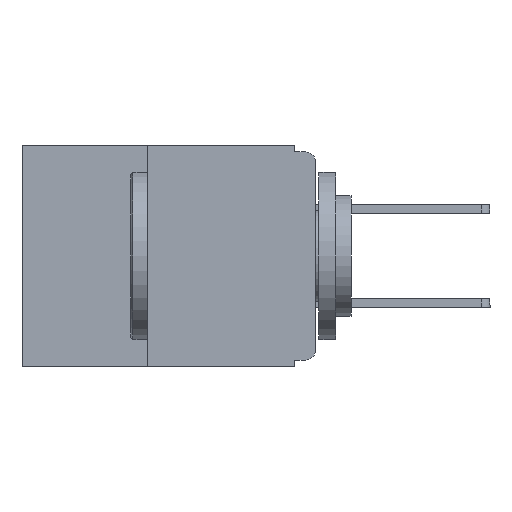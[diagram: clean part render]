
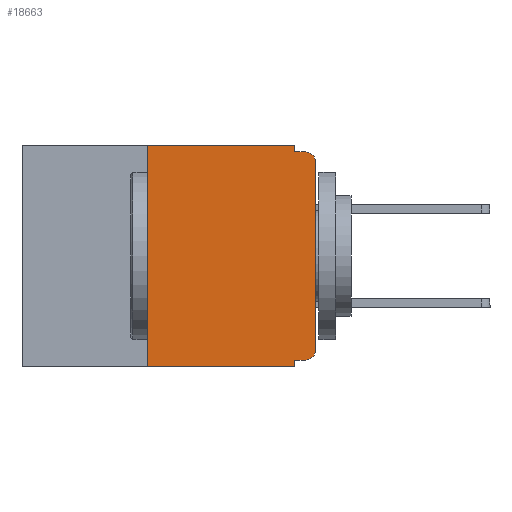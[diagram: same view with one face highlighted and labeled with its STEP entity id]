
A CAD part, left-side view. The second image highlights one B-rep face of the part: STEP entity #18663.
In plain terms, the highlighted planar face has unit normal (-1, 0, 0).
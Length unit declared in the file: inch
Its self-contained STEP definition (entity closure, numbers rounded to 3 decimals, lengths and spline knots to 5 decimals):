
#309 = EDGE_CURVE ( 'NONE', #14362, #420, #9314, .T. ) ;
#420 = VERTEX_POINT ( 'NONE', #20970 ) ;
#1340 = EDGE_CURVE ( 'NONE', #6322, #14299, #17589, .T. ) ;
#1489 = VERTEX_POINT ( 'NONE', #14184 ) ;
#2234 = ORIENTED_EDGE ( 'NONE', *, *, #12778, .T. ) ;
#2602 = ORIENTED_EDGE ( 'NONE', *, *, #5748, .F. ) ;
#2698 = ORIENTED_EDGE ( 'NONE', *, *, #8551, .T. ) ;
#2961 = CARTESIAN_POINT ( 'NONE',  ( 0., 0., -0.01 ) ) ;
#3561 = CARTESIAN_POINT ( 'NONE',  ( 0., 0.031, -0.01 ) ) ;
#3616 = VECTOR ( 'NONE', #21447, 39.37008 ) ;
#3746 = VERTEX_POINT ( 'NONE', #11124 ) ;
#4279 = ORIENTED_EDGE ( 'NONE', *, *, #15386, .T. ) ;
#4288 = ORIENTED_EDGE ( 'NONE', *, *, #10600, .F. ) ;
#4290 = LINE ( 'NONE', #2961, #12814 ) ;
#4344 = CARTESIAN_POINT ( 'NONE',  ( 0., 0., -0.32 ) ) ;
#4384 = DIRECTION ( 'NONE',  ( 0., 0., -1. ) ) ;
#4617 = VERTEX_POINT ( 'NONE', #19635 ) ;
#4708 = DIRECTION ( 'NONE',  ( 0., -1., 0. ) ) ;
#5220 = DIRECTION ( 'NONE',  ( 0., -1., 0. ) ) ;
#5565 = VECTOR ( 'NONE', #5220, 39.37008 ) ;
#5639 = DIRECTION ( 'NONE',  ( 0., 1., 0. ) ) ;
#5748 = EDGE_CURVE ( 'NONE', #3746, #12291, #14736, .T. ) ;
#6243 = DIRECTION ( 'NONE',  ( 0., 0., 1. ) ) ;
#6317 = PLANE ( 'NONE',  #16685 ) ;
#6322 = VERTEX_POINT ( 'NONE', #11611 ) ;
#6332 = CARTESIAN_POINT ( 'NONE',  ( 0., 0., 0. ) ) ;
#6452 = DIRECTION ( 'NONE',  ( 0., -1., 0. ) ) ;
#6865 = LINE ( 'NONE', #4344, #11410 ) ;
#7360 = EDGE_LOOP ( 'NONE', ( #2234, #2698, #13520, #14087, #4288, #2602, #4279, #10734, #19033, #18287 ) ) ;
#8551 = EDGE_CURVE ( 'NONE', #4617, #1489, #9394, .T. ) ;
#8654 = CARTESIAN_POINT ( 'NONE',  ( 0., 0.031, 0. ) ) ;
#9064 = LINE ( 'NONE', #8654, #17898 ) ;
#9314 = CIRCLE ( 'NONE', #10658, 0.015 ) ;
#9394 = CIRCLE ( 'NONE', #10488, 0.015 ) ;
#9751 = DIRECTION ( 'NONE',  ( 1., 0., 0. ) ) ;
#10041 = CARTESIAN_POINT ( 'NONE',  ( 0., 0.031, -0.33 ) ) ;
#10049 = VERTEX_POINT ( 'NONE', #3561 ) ;
#10380 = DIRECTION ( 'NONE',  ( 0., 0., -1. ) ) ;
#10488 = AXIS2_PLACEMENT_3D ( 'NONE', #18037, #18027, #17991 ) ;
#10600 = EDGE_CURVE ( 'NONE', #12291, #19968, #15083, .T. ) ;
#10658 = AXIS2_PLACEMENT_3D ( 'NONE', #21500, #12845, #4384 ) ;
#10734 = ORIENTED_EDGE ( 'NONE', *, *, #1340, .F. ) ;
#11124 = CARTESIAN_POINT ( 'NONE',  ( 0., 0.25, -0.33 ) ) ;
#11225 = EDGE_CURVE ( 'NONE', #14362, #6322, #6865, .T. ) ;
#11379 = VECTOR ( 'NONE', #6243, 39.37008 ) ;
#11410 = VECTOR ( 'NONE', #5639, 39.37008 ) ;
#11588 = CARTESIAN_POINT ( 'NONE',  ( 0., 0.25, 0. ) ) ;
#11611 = CARTESIAN_POINT ( 'NONE',  ( 0., 0.031, -0.32 ) ) ;
#11764 = VECTOR ( 'NONE', #6452, 39.37008 ) ;
#11915 = FACE_OUTER_BOUND ( 'NONE', #7360, .T. ) ;
#12291 = VERTEX_POINT ( 'NONE', #11588 ) ;
#12778 = EDGE_CURVE ( 'NONE', #420, #4617, #15812, .T. ) ;
#12814 = VECTOR ( 'NONE', #4708, 39.37008 ) ;
#12845 = DIRECTION ( 'NONE',  ( -1., 0., 0. ) ) ;
#13343 = CARTESIAN_POINT ( 'NONE',  ( 0., 0.437, -0.33 ) ) ;
#13520 = ORIENTED_EDGE ( 'NONE', *, *, #15347, .F. ) ;
#14087 = ORIENTED_EDGE ( 'NONE', *, *, #17657, .F. ) ;
#14184 = CARTESIAN_POINT ( 'NONE',  ( 0., 0.015, -0.01 ) ) ;
#14299 = VERTEX_POINT ( 'NONE', #20276 ) ;
#14362 = VERTEX_POINT ( 'NONE', #15627 ) ;
#14391 = CARTESIAN_POINT ( 'NONE',  ( 0., 0.031, 0. ) ) ;
#14736 = LINE ( 'NONE', #17342, #18551 ) ;
#15083 = LINE ( 'NONE', #15618, #5565 ) ;
#15347 = EDGE_CURVE ( 'NONE', #10049, #1489, #4290, .T. ) ;
#15386 = EDGE_CURVE ( 'NONE', #3746, #14299, #21446, .T. ) ;
#15618 = CARTESIAN_POINT ( 'NONE',  ( 0., 0.437, 0. ) ) ;
#15627 = CARTESIAN_POINT ( 'NONE',  ( 0., 0.015, -0.32 ) ) ;
#15812 = LINE ( 'NONE', #6332, #11379 ) ;
#16685 = AXIS2_PLACEMENT_3D ( 'NONE', #18002, #9751, #21202 ) ;
#17342 = CARTESIAN_POINT ( 'NONE',  ( 0., 0.25, -0.33 ) ) ;
#17365 = DIRECTION ( 'NONE',  ( 0., 0., 1. ) ) ;
#17589 = LINE ( 'NONE', #10041, #3616 ) ;
#17657 = EDGE_CURVE ( 'NONE', #19968, #10049, #9064, .T. ) ;
#17898 = VECTOR ( 'NONE', #10380, 39.37008 ) ;
#17991 = DIRECTION ( 'NONE',  ( 0., 0., -1. ) ) ;
#18002 = CARTESIAN_POINT ( 'NONE',  ( 0., 0.437, 0. ) ) ;
#18027 = DIRECTION ( 'NONE',  ( -1., 0., 0. ) ) ;
#18037 = CARTESIAN_POINT ( 'NONE',  ( 0., 0.015, -0.025 ) ) ;
#18287 = ORIENTED_EDGE ( 'NONE', *, *, #309, .T. ) ;
#18551 = VECTOR ( 'NONE', #17365, 39.37008 ) ;
#18663 = ADVANCED_FACE ( 'NONE', ( #11915 ), #6317, .F. ) ;
#19033 = ORIENTED_EDGE ( 'NONE', *, *, #11225, .F. ) ;
#19635 = CARTESIAN_POINT ( 'NONE',  ( 0., 0., -0.025 ) ) ;
#19968 = VERTEX_POINT ( 'NONE', #14391 ) ;
#20276 = CARTESIAN_POINT ( 'NONE',  ( 0., 0.031, -0.33 ) ) ;
#20970 = CARTESIAN_POINT ( 'NONE',  ( 0., 0., -0.305 ) ) ;
#21202 = DIRECTION ( 'NONE',  ( 0., 0., -1. ) ) ;
#21446 = LINE ( 'NONE', #13343, #11764 ) ;
#21447 = DIRECTION ( 'NONE',  ( 0., 0., -1. ) ) ;
#21500 = CARTESIAN_POINT ( 'NONE',  ( 0., 0.015, -0.305 ) ) ;
